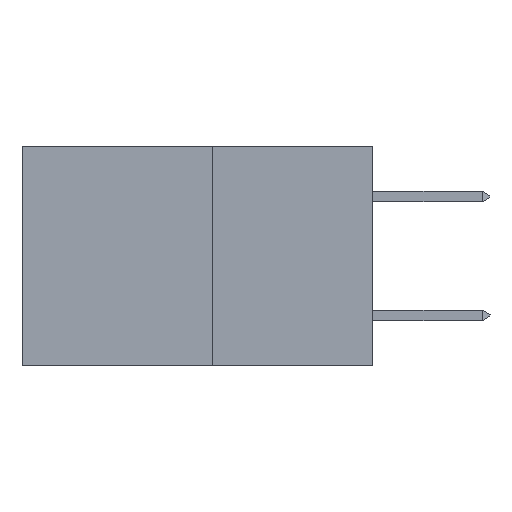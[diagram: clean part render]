
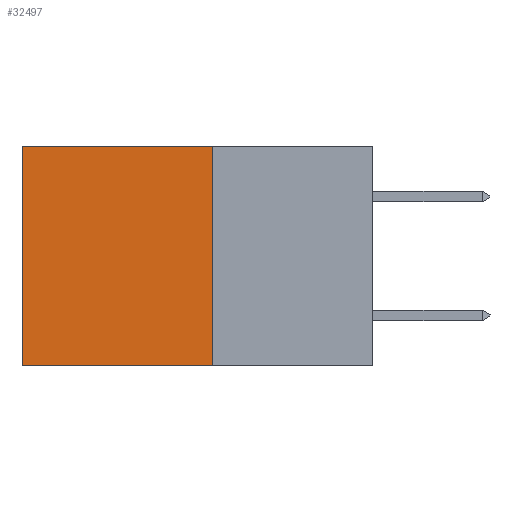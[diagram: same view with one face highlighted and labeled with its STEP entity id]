
A CAD part, left-side view. The second image highlights one B-rep face of the part: STEP entity #32497.
In plain terms, the highlighted planar face has unit normal (-1, 0, 0).
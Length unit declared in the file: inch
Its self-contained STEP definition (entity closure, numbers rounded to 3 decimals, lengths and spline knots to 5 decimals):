
#659 = DIRECTION ( 'NONE',  ( 0., 1., 0. ) ) ;
#1199 = DIRECTION ( 'NONE',  ( 0., 1., 0. ) ) ;
#1379 = ORIENTED_EDGE ( 'NONE', *, *, #14232, .T. ) ;
#1869 = CARTESIAN_POINT ( 'NONE',  ( 0.277, 0.27, -0.37 ) ) ;
#2670 = LINE ( 'NONE', #23541, #7956 ) ;
#3076 = EDGE_CURVE ( 'NONE', #3784, #12062, #26254, .T. ) ;
#3784 = VERTEX_POINT ( 'NONE', #8606 ) ;
#5749 = EDGE_CURVE ( 'NONE', #12062, #20749, #2670, .T. ) ;
#6294 = CARTESIAN_POINT ( 'NONE',  ( 0.277, 0.27, 0. ) ) ;
#6601 = CARTESIAN_POINT ( 'NONE',  ( 0.277, 0.59, -0.37 ) ) ;
#6716 = VECTOR ( 'NONE', #19339, 39.37008 ) ;
#7956 = VECTOR ( 'NONE', #659, 39.37008 ) ;
#8606 = CARTESIAN_POINT ( 'NONE',  ( 0.277, 0.27, 0. ) ) ;
#12032 = ORIENTED_EDGE ( 'NONE', *, *, #12820, .T. ) ;
#12062 = VERTEX_POINT ( 'NONE', #28240 ) ;
#12250 = DIRECTION ( 'NONE',  ( 1., 0., 0. ) ) ;
#12820 = EDGE_CURVE ( 'NONE', #3784, #28459, #13642, .T. ) ;
#13642 = LINE ( 'NONE', #6294, #26207 ) ;
#14232 = EDGE_CURVE ( 'NONE', #28459, #20749, #20287, .T. ) ;
#17805 = CARTESIAN_POINT ( 'NONE',  ( 0.277, 0.59, 0. ) ) ;
#19339 = DIRECTION ( 'NONE',  ( 0., 0., -1. ) ) ;
#19687 = AXIS2_PLACEMENT_3D ( 'NONE', #1869, #12250, #29843 ) ;
#20287 = LINE ( 'NONE', #6601, #6716 ) ;
#20749 = VERTEX_POINT ( 'NONE', #22304 ) ;
#21792 = EDGE_LOOP ( 'NONE', ( #1379, #22945, #31599, #12032 ) ) ;
#22304 = CARTESIAN_POINT ( 'NONE',  ( 0.277, 0.59, -0.37 ) ) ;
#22310 = PLANE ( 'NONE',  #19687 ) ;
#22945 = ORIENTED_EDGE ( 'NONE', *, *, #5749, .F. ) ;
#23541 = CARTESIAN_POINT ( 'NONE',  ( 0.277, 0.27, -0.37 ) ) ;
#25086 = CARTESIAN_POINT ( 'NONE',  ( 0.277, 0.27, -0.37 ) ) ;
#25163 = DIRECTION ( 'NONE',  ( 0., 0., -1. ) ) ;
#25495 = FACE_OUTER_BOUND ( 'NONE', #21792, .T. ) ;
#26207 = VECTOR ( 'NONE', #1199, 39.37008 ) ;
#26254 = LINE ( 'NONE', #25086, #32153 ) ;
#28240 = CARTESIAN_POINT ( 'NONE',  ( 0.277, 0.27, -0.37 ) ) ;
#28459 = VERTEX_POINT ( 'NONE', #17805 ) ;
#29843 = DIRECTION ( 'NONE',  ( 0., 0., -1. ) ) ;
#31599 = ORIENTED_EDGE ( 'NONE', *, *, #3076, .F. ) ;
#32153 = VECTOR ( 'NONE', #25163, 39.37008 ) ;
#32497 = ADVANCED_FACE ( 'NONE', ( #25495 ), #22310, .F. ) ;
